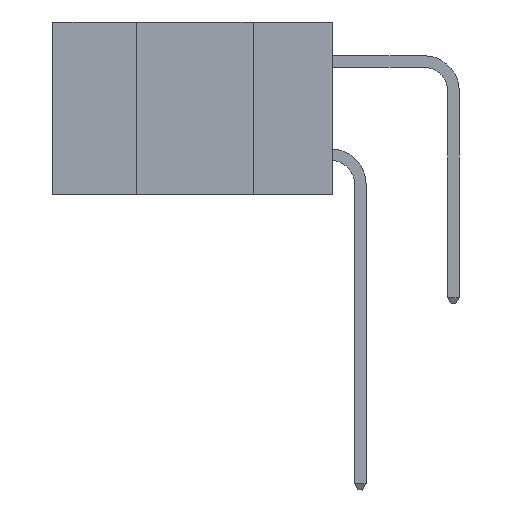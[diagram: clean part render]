
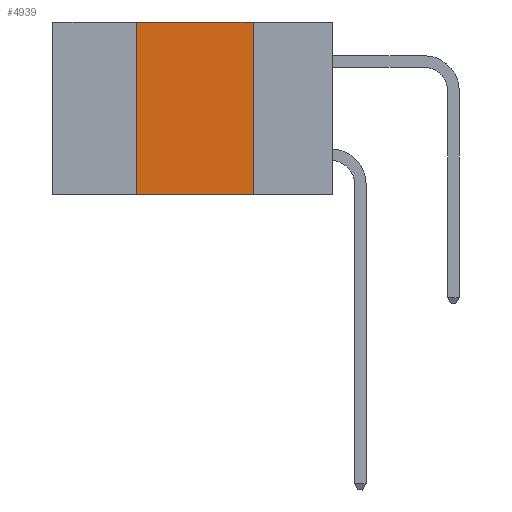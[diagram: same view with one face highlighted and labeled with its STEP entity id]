
A CAD part, left-side view. The second image highlights one B-rep face of the part: STEP entity #4939.
In plain terms, the highlighted planar face has unit normal (-1, 0, 0).
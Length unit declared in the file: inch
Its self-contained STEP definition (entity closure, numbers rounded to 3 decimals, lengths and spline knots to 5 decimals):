
#447 = CARTESIAN_POINT ( 'NONE',  ( 0., 0.6, 0. ) ) ;
#584 = CARTESIAN_POINT ( 'NONE',  ( 0., 0.17, -0.37 ) ) ;
#1203 = LINE ( 'NONE', #6242, #8705 ) ;
#1598 = DIRECTION ( 'NONE',  ( 0., 0., -1. ) ) ;
#1644 = EDGE_LOOP ( 'NONE', ( #3010, #14831, #14629, #7555 ) ) ;
#1715 = VECTOR ( 'NONE', #13981, 39.37008 ) ;
#1987 = DIRECTION ( 'NONE',  ( 0., 0., -1. ) ) ;
#2034 = VERTEX_POINT ( 'NONE', #13766 ) ;
#2587 = CARTESIAN_POINT ( 'NONE',  ( 0., 0.42, -0.37 ) ) ;
#3010 = ORIENTED_EDGE ( 'NONE', *, *, #8636, .F. ) ;
#4939 = ADVANCED_FACE ( 'NONE', ( #10405 ), #13906, .F. ) ;
#5838 = CARTESIAN_POINT ( 'NONE',  ( 0., 0.42, -0.37 ) ) ;
#6242 = CARTESIAN_POINT ( 'NONE',  ( 0., 0.6, 0. ) ) ;
#6547 = EDGE_CURVE ( 'NONE', #10099, #13184, #14131, .T. ) ;
#7283 = VERTEX_POINT ( 'NONE', #9384 ) ;
#7555 = ORIENTED_EDGE ( 'NONE', *, *, #10259, .T. ) ;
#7639 = VECTOR ( 'NONE', #1987, 39.37008 ) ;
#7641 = DIRECTION ( 'NONE',  ( 1., 0., 0. ) ) ;
#8619 = CARTESIAN_POINT ( 'NONE',  ( 0., 0.6, -0.37 ) ) ;
#8636 = EDGE_CURVE ( 'NONE', #2034, #7283, #10902, .T. ) ;
#8705 = VECTOR ( 'NONE', #11280, 39.37008 ) ;
#9384 = CARTESIAN_POINT ( 'NONE',  ( 0., 0.17, -0.37 ) ) ;
#10099 = VERTEX_POINT ( 'NONE', #5838 ) ;
#10259 = EDGE_CURVE ( 'NONE', #10099, #7283, #12675, .T. ) ;
#10405 = FACE_OUTER_BOUND ( 'NONE', #1644, .T. ) ;
#10902 = LINE ( 'NONE', #584, #7639 ) ;
#11280 = DIRECTION ( 'NONE',  ( 0., -1., 0. ) ) ;
#11343 = CARTESIAN_POINT ( 'NONE',  ( 0., 0.42, 0. ) ) ;
#12675 = LINE ( 'NONE', #8619, #16025 ) ;
#13184 = VERTEX_POINT ( 'NONE', #11343 ) ;
#13766 = CARTESIAN_POINT ( 'NONE',  ( 0., 0.17, 0. ) ) ;
#13906 = PLANE ( 'NONE',  #15275 ) ;
#13911 = DIRECTION ( 'NONE',  ( 0., -1., 0. ) ) ;
#13981 = DIRECTION ( 'NONE',  ( 0., 0., 1. ) ) ;
#14131 = LINE ( 'NONE', #2587, #1715 ) ;
#14629 = ORIENTED_EDGE ( 'NONE', *, *, #6547, .F. ) ;
#14831 = ORIENTED_EDGE ( 'NONE', *, *, #16043, .F. ) ;
#15275 = AXIS2_PLACEMENT_3D ( 'NONE', #447, #7641, #1598 ) ;
#16025 = VECTOR ( 'NONE', #13911, 39.37008 ) ;
#16043 = EDGE_CURVE ( 'NONE', #13184, #2034, #1203, .T. ) ;
